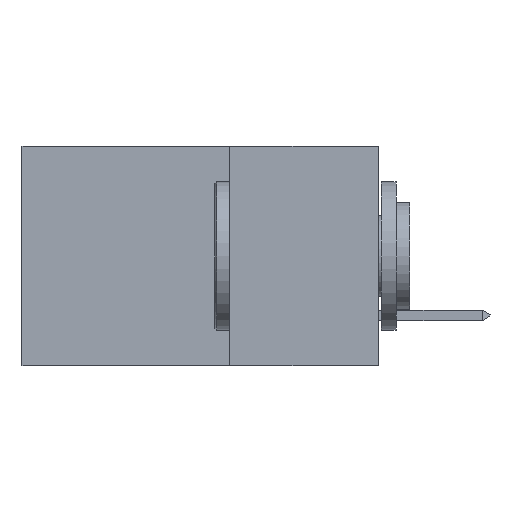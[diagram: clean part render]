
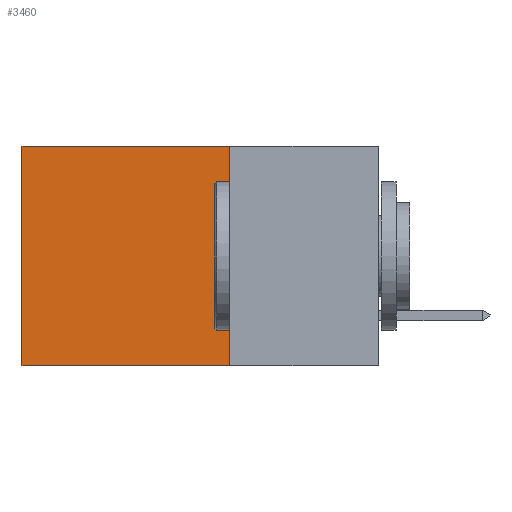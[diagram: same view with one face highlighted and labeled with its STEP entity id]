
A CAD part, left-side view. The second image highlights one B-rep face of the part: STEP entity #3460.
In plain terms, the highlighted planar face has unit normal (-1, 0, 0).
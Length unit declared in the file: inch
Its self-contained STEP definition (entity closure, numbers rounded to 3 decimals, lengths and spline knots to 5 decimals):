
#139 = EDGE_CURVE ( 'NONE', #15320, #6692, #14439, .T. ) ;
#780 = DIRECTION ( 'NONE',  ( 1., 0., 0. ) ) ;
#1072 = DIRECTION ( 'NONE',  ( 0., 1., 0. ) ) ;
#1430 = VECTOR ( 'NONE', #9461, 39.37008 ) ;
#3259 = PLANE ( 'NONE',  #4728 ) ;
#3460 = ADVANCED_FACE ( 'NONE', ( #7210 ), #3259, .F. ) ;
#4042 = CARTESIAN_POINT ( 'NONE',  ( 0.2615, 0.25, -0.37 ) ) ;
#4592 = CARTESIAN_POINT ( 'NONE',  ( 0.2615, 0.25, -0.37 ) ) ;
#4725 = CARTESIAN_POINT ( 'NONE',  ( 0.2615, 0.6, -0.37 ) ) ;
#4728 = AXIS2_PLACEMENT_3D ( 'NONE', #4592, #780, #16810 ) ;
#4859 = VERTEX_POINT ( 'NONE', #9186 ) ;
#5063 = VECTOR ( 'NONE', #8341, 39.37008 ) ;
#5971 = EDGE_CURVE ( 'NONE', #16264, #6692, #15387, .T. ) ;
#6692 = VERTEX_POINT ( 'NONE', #14397 ) ;
#6931 = ORIENTED_EDGE ( 'NONE', *, *, #5971, .T. ) ;
#7210 = FACE_OUTER_BOUND ( 'NONE', #11013, .T. ) ;
#7565 = EDGE_CURVE ( 'NONE', #4859, #15320, #8070, .T. ) ;
#7757 = LINE ( 'NONE', #11600, #10800 ) ;
#8070 = LINE ( 'NONE', #4042, #1430 ) ;
#8341 = DIRECTION ( 'NONE',  ( 0., 0., -1. ) ) ;
#9186 = CARTESIAN_POINT ( 'NONE',  ( 0.2615, 0.25, 0. ) ) ;
#9461 = DIRECTION ( 'NONE',  ( 0., 0., -1. ) ) ;
#9494 = VECTOR ( 'NONE', #13306, 39.37008 ) ;
#10800 = VECTOR ( 'NONE', #1072, 39.37008 ) ;
#11013 = EDGE_LOOP ( 'NONE', ( #6931, #16045, #15679, #13132 ) ) ;
#11600 = CARTESIAN_POINT ( 'NONE',  ( 0.2615, 0.25, 0. ) ) ;
#13132 = ORIENTED_EDGE ( 'NONE', *, *, #14567, .T. ) ;
#13219 = CARTESIAN_POINT ( 'NONE',  ( 0.2615, 0.25, -0.37 ) ) ;
#13306 = DIRECTION ( 'NONE',  ( 0., 1., 0. ) ) ;
#14397 = CARTESIAN_POINT ( 'NONE',  ( 0.2615, 0.6, -0.37 ) ) ;
#14439 = LINE ( 'NONE', #13219, #9494 ) ;
#14567 = EDGE_CURVE ( 'NONE', #4859, #16264, #7757, .T. ) ;
#14973 = CARTESIAN_POINT ( 'NONE',  ( 0.2615, 0.25, -0.37 ) ) ;
#15320 = VERTEX_POINT ( 'NONE', #14973 ) ;
#15387 = LINE ( 'NONE', #4725, #5063 ) ;
#15679 = ORIENTED_EDGE ( 'NONE', *, *, #7565, .F. ) ;
#16045 = ORIENTED_EDGE ( 'NONE', *, *, #139, .F. ) ;
#16264 = VERTEX_POINT ( 'NONE', #17074 ) ;
#16810 = DIRECTION ( 'NONE',  ( 0., 0., -1. ) ) ;
#17074 = CARTESIAN_POINT ( 'NONE',  ( 0.2615, 0.6, 0. ) ) ;
